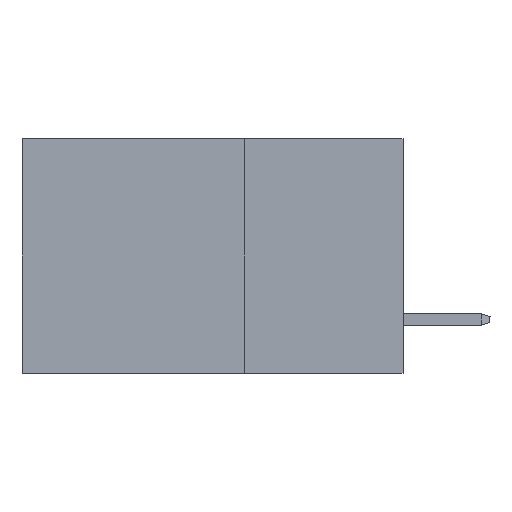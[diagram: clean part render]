
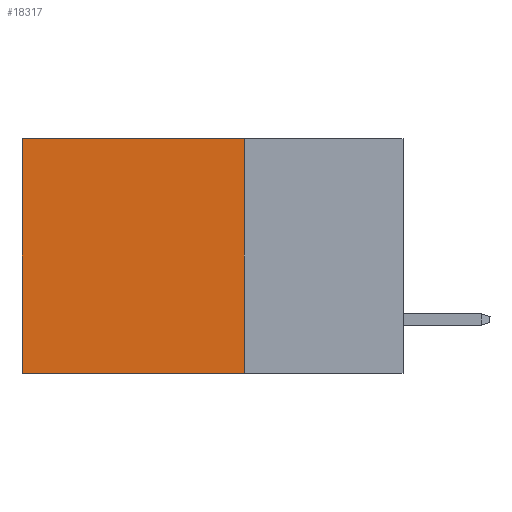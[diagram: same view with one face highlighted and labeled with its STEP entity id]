
A CAD part, left-side view. The second image highlights one B-rep face of the part: STEP entity #18317.
In plain terms, the highlighted planar face has unit normal (-1, 0, 0).
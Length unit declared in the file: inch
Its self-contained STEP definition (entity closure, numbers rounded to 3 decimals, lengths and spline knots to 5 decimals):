
#397 = AXIS2_PLACEMENT_3D ( 'NONE', #26642, #26422, #12204 ) ;
#1406 = ORIENTED_EDGE ( 'NONE', *, *, #17795, .T. ) ;
#1875 = VECTOR ( 'NONE', #8478, 39.37008 ) ;
#2294 = PLANE ( 'NONE',  #397 ) ;
#3893 = VERTEX_POINT ( 'NONE', #19795 ) ;
#5444 = CARTESIAN_POINT ( 'NONE',  ( 0.2875, 0.25, 0. ) ) ;
#6239 = CARTESIAN_POINT ( 'NONE',  ( 0.2875, 0.25, 0. ) ) ;
#7605 = VERTEX_POINT ( 'NONE', #39070 ) ;
#8478 = DIRECTION ( 'NONE',  ( 0., 0., -1. ) ) ;
#9635 = LINE ( 'NONE', #6239, #40789 ) ;
#11983 = FACE_OUTER_BOUND ( 'NONE', #15661, .T. ) ;
#12204 = DIRECTION ( 'NONE',  ( 0., 0., -1. ) ) ;
#12297 = VERTEX_POINT ( 'NONE', #5444 ) ;
#13109 = ORIENTED_EDGE ( 'NONE', *, *, #42901, .T. ) ;
#15661 = EDGE_LOOP ( 'NONE', ( #1406, #43311, #41897, #13109 ) ) ;
#16472 = VERTEX_POINT ( 'NONE', #27492 ) ;
#17795 = EDGE_CURVE ( 'NONE', #7605, #16472, #35352, .T. ) ;
#18317 = ADVANCED_FACE ( 'NONE', ( #11983 ), #2294, .F. ) ;
#19795 = CARTESIAN_POINT ( 'NONE',  ( 0.2875, 0.25, -0.37 ) ) ;
#25364 = CARTESIAN_POINT ( 'NONE',  ( 0.2875, 0.6, 0. ) ) ;
#26422 = DIRECTION ( 'NONE',  ( 1., 0., 0. ) ) ;
#26642 = CARTESIAN_POINT ( 'NONE',  ( 0.2875, 0.25, 0. ) ) ;
#27492 = CARTESIAN_POINT ( 'NONE',  ( 0.2875, 0.6, -0.37 ) ) ;
#35146 = DIRECTION ( 'NONE',  ( 0., 0., -1. ) ) ;
#35352 = LINE ( 'NONE', #25364, #42193 ) ;
#37043 = EDGE_CURVE ( 'NONE', #3893, #16472, #37170, .T. ) ;
#37170 = LINE ( 'NONE', #40984, #41978 ) ;
#37604 = DIRECTION ( 'NONE',  ( 0., 1., 0. ) ) ;
#39070 = CARTESIAN_POINT ( 'NONE',  ( 0.2875, 0.6, 0. ) ) ;
#39648 = LINE ( 'NONE', #42835, #1875 ) ;
#40789 = VECTOR ( 'NONE', #44206, 39.37008 ) ;
#40984 = CARTESIAN_POINT ( 'NONE',  ( 0.2875, 0.25, -0.37 ) ) ;
#41897 = ORIENTED_EDGE ( 'NONE', *, *, #42560, .F. ) ;
#41978 = VECTOR ( 'NONE', #37604, 39.37008 ) ;
#42193 = VECTOR ( 'NONE', #35146, 39.37008 ) ;
#42560 = EDGE_CURVE ( 'NONE', #12297, #3893, #39648, .T. ) ;
#42835 = CARTESIAN_POINT ( 'NONE',  ( 0.2875, 0.25, 0. ) ) ;
#42901 = EDGE_CURVE ( 'NONE', #12297, #7605, #9635, .T. ) ;
#43311 = ORIENTED_EDGE ( 'NONE', *, *, #37043, .F. ) ;
#44206 = DIRECTION ( 'NONE',  ( 0., 1., 0. ) ) ;
